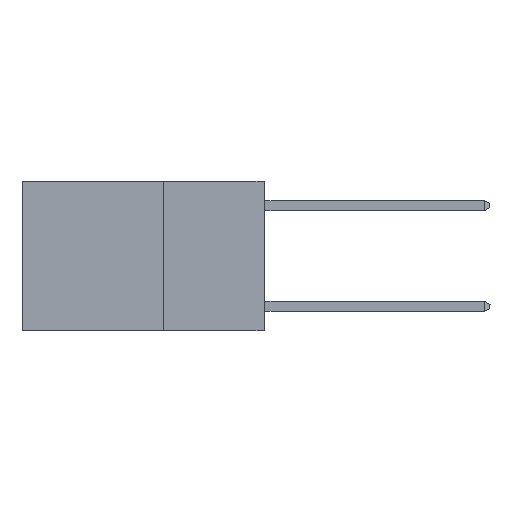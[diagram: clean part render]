
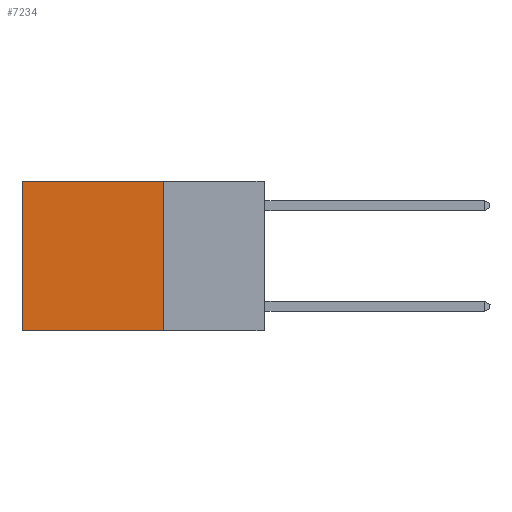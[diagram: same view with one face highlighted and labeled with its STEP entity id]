
A CAD part, left-side view. The second image highlights one B-rep face of the part: STEP entity #7234.
In plain terms, the highlighted planar face has unit normal (-1, 0, 0).
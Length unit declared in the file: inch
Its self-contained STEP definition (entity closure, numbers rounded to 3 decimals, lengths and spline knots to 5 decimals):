
#501 = VERTEX_POINT ( 'NONE', #14393 ) ;
#605 = LINE ( 'NONE', #17107, #18563 ) ;
#804 = DIRECTION ( 'NONE',  ( 0., 0., -1. ) ) ;
#1395 = DIRECTION ( 'NONE',  ( 0., 1., 0. ) ) ;
#2018 = EDGE_CURVE ( 'NONE', #14778, #14155, #6045, .T. ) ;
#3480 = ORIENTED_EDGE ( 'NONE', *, *, #2018, .T. ) ;
#3905 = CARTESIAN_POINT ( 'NONE',  ( 0.2625, 0.25, -0.37 ) ) ;
#5973 = VECTOR ( 'NONE', #14354, 39.37008 ) ;
#6045 = LINE ( 'NONE', #6252, #14772 ) ;
#6252 = CARTESIAN_POINT ( 'NONE',  ( 0.2625, 0.6, 0. ) ) ;
#6680 = DIRECTION ( 'NONE',  ( 1., 0., 0. ) ) ;
#6745 = AXIS2_PLACEMENT_3D ( 'NONE', #15344, #6680, #18768 ) ;
#6763 = CARTESIAN_POINT ( 'NONE',  ( 0.2625, 0.25, -0.37 ) ) ;
#7234 = ADVANCED_FACE ( 'NONE', ( #9580 ), #22116, .F. ) ;
#7342 = LINE ( 'NONE', #13073, #20552 ) ;
#8048 = EDGE_CURVE ( 'NONE', #17293, #14155, #15222, .T. ) ;
#8213 = EDGE_CURVE ( 'NONE', #501, #17293, #7342, .T. ) ;
#8480 = ORIENTED_EDGE ( 'NONE', *, *, #13382, .T. ) ;
#9580 = FACE_OUTER_BOUND ( 'NONE', #19862, .T. ) ;
#11356 = ORIENTED_EDGE ( 'NONE', *, *, #8213, .F. ) ;
#12414 = CARTESIAN_POINT ( 'NONE',  ( 0.2625, 0.6, 0. ) ) ;
#13073 = CARTESIAN_POINT ( 'NONE',  ( 0.2625, 0.25, 0. ) ) ;
#13382 = EDGE_CURVE ( 'NONE', #501, #14778, #605, .T. ) ;
#14155 = VERTEX_POINT ( 'NONE', #20718 ) ;
#14354 = DIRECTION ( 'NONE',  ( 0., 1., 0. ) ) ;
#14385 = ORIENTED_EDGE ( 'NONE', *, *, #8048, .F. ) ;
#14393 = CARTESIAN_POINT ( 'NONE',  ( 0.2625, 0.25, 0. ) ) ;
#14772 = VECTOR ( 'NONE', #20072, 39.37008 ) ;
#14778 = VERTEX_POINT ( 'NONE', #12414 ) ;
#15222 = LINE ( 'NONE', #3905, #5973 ) ;
#15344 = CARTESIAN_POINT ( 'NONE',  ( 0.2625, 0.25, 0. ) ) ;
#17107 = CARTESIAN_POINT ( 'NONE',  ( 0.2625, 0.25, 0. ) ) ;
#17293 = VERTEX_POINT ( 'NONE', #6763 ) ;
#18563 = VECTOR ( 'NONE', #1395, 39.37008 ) ;
#18768 = DIRECTION ( 'NONE',  ( 0., 0., -1. ) ) ;
#19862 = EDGE_LOOP ( 'NONE', ( #3480, #14385, #11356, #8480 ) ) ;
#20072 = DIRECTION ( 'NONE',  ( 0., 0., -1. ) ) ;
#20552 = VECTOR ( 'NONE', #804, 39.37008 ) ;
#20718 = CARTESIAN_POINT ( 'NONE',  ( 0.2625, 0.6, -0.37 ) ) ;
#22116 = PLANE ( 'NONE',  #6745 ) ;
